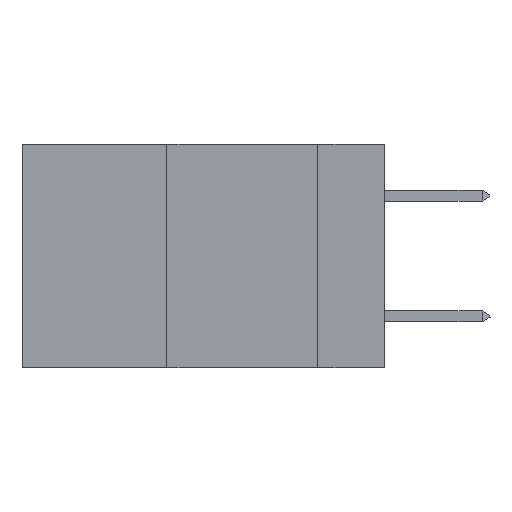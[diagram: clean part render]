
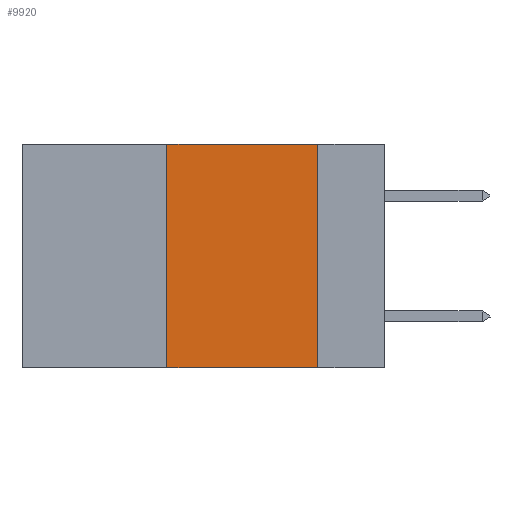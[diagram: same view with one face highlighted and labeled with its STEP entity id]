
A CAD part, left-side view. The second image highlights one B-rep face of the part: STEP entity #9920.
In plain terms, the highlighted planar face has unit normal (-1, 0, 0).
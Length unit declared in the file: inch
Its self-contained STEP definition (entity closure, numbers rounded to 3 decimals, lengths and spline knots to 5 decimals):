
#11 = VERTEX_POINT ( 'NONE', #1740 ) ;
#351 = ORIENTED_EDGE ( 'NONE', *, *, #2624, .F. ) ;
#382 = CARTESIAN_POINT ( 'NONE',  ( 0., 0.6, 0. ) ) ;
#1163 = ORIENTED_EDGE ( 'NONE', *, *, #10346, .F. ) ;
#1206 = DIRECTION ( 'NONE',  ( 0., 0., -1. ) ) ;
#1298 = CARTESIAN_POINT ( 'NONE',  ( 0., 0.6, 0. ) ) ;
#1521 = LINE ( 'NONE', #1298, #7141 ) ;
#1740 = CARTESIAN_POINT ( 'NONE',  ( 0., 0.36, 0. ) ) ;
#1913 = LINE ( 'NONE', #3496, #4550 ) ;
#2624 = EDGE_CURVE ( 'NONE', #11, #3130, #1521, .T. ) ;
#2801 = PLANE ( 'NONE',  #3502 ) ;
#3112 = DIRECTION ( 'NONE',  ( 0., 0., -1. ) ) ;
#3130 = VERTEX_POINT ( 'NONE', #5913 ) ;
#3496 = CARTESIAN_POINT ( 'NONE',  ( 0., 0.36, 0. ) ) ;
#3502 = AXIS2_PLACEMENT_3D ( 'NONE', #382, #9238, #1206 ) ;
#3776 = DIRECTION ( 'NONE',  ( 0., -1., 0. ) ) ;
#3918 = ORIENTED_EDGE ( 'NONE', *, *, #8843, .F. ) ;
#4311 = FACE_OUTER_BOUND ( 'NONE', #7701, .T. ) ;
#4550 = VECTOR ( 'NONE', #5905, 39.37008 ) ;
#5059 = LINE ( 'NONE', #7073, #6309 ) ;
#5249 = EDGE_CURVE ( 'NONE', #5588, #7087, #8957, .T. ) ;
#5408 = CARTESIAN_POINT ( 'NONE',  ( 0., 0.6, -0.37 ) ) ;
#5588 = VERTEX_POINT ( 'NONE', #9922 ) ;
#5905 = DIRECTION ( 'NONE',  ( 0., 0., 1. ) ) ;
#5913 = CARTESIAN_POINT ( 'NONE',  ( 0., 0.11, 0. ) ) ;
#6034 = ORIENTED_EDGE ( 'NONE', *, *, #5249, .T. ) ;
#6309 = VECTOR ( 'NONE', #3112, 39.37008 ) ;
#6479 = CARTESIAN_POINT ( 'NONE',  ( 0., 0.11, -0.37 ) ) ;
#7073 = CARTESIAN_POINT ( 'NONE',  ( 0., 0.11, 0. ) ) ;
#7087 = VERTEX_POINT ( 'NONE', #6479 ) ;
#7141 = VECTOR ( 'NONE', #3776, 39.37008 ) ;
#7701 = EDGE_LOOP ( 'NONE', ( #3918, #351, #1163, #6034 ) ) ;
#8680 = DIRECTION ( 'NONE',  ( 0., -1., 0. ) ) ;
#8843 = EDGE_CURVE ( 'NONE', #3130, #7087, #5059, .T. ) ;
#8851 = VECTOR ( 'NONE', #8680, 39.37008 ) ;
#8957 = LINE ( 'NONE', #5408, #8851 ) ;
#9238 = DIRECTION ( 'NONE',  ( 1., 0., 0. ) ) ;
#9920 = ADVANCED_FACE ( 'NONE', ( #4311 ), #2801, .F. ) ;
#9922 = CARTESIAN_POINT ( 'NONE',  ( 0., 0.36, -0.37 ) ) ;
#10346 = EDGE_CURVE ( 'NONE', #5588, #11, #1913, .T. ) ;
